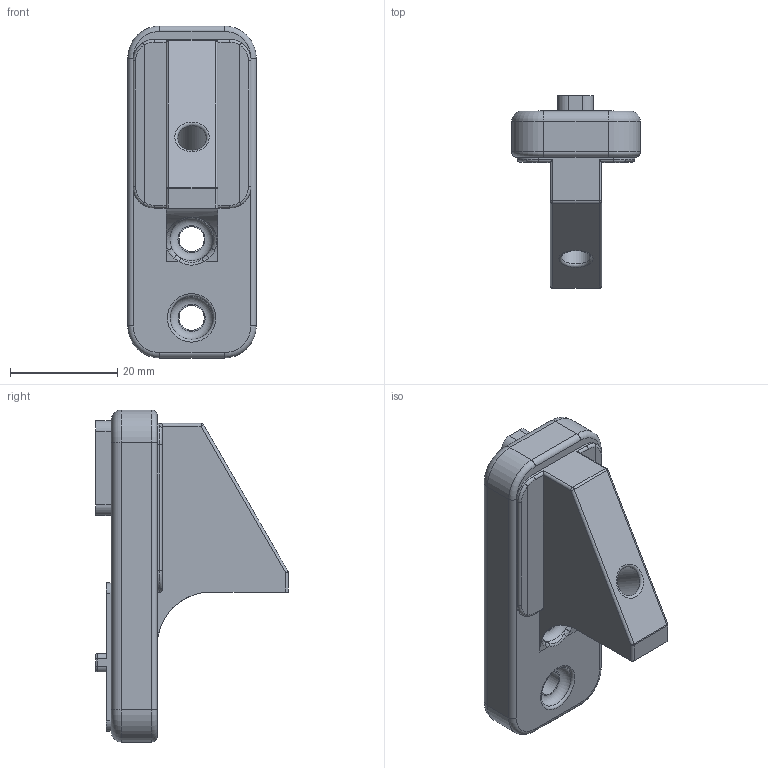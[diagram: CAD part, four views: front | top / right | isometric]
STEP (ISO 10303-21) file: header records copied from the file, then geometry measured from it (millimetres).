
FILE_DESCRIPTION(/* description */ (''),/* implementation_level */ '2;1');
FILE_NAME(/* name */ 'foregrip-adapter-mlok-freeman1337.step',/* time_stamp */ '2021-04-15T20:24:15-07:00',/* author */ (''),/* organization */ (''),/* preprocessor_version */ 'ST-DEVELOPER v18.1',/* originating_system */ 'Autodesk Translation Framework v10.6.0.1341',/* authorisation */ '');
FILE_SCHEMA (('AUTOMOTIVE_DESIGN { 1 0 10303 214 3 1 1 }'));
Length unit declared in the file: millimetre
Products named in the file (1): mlok-adapter
Bounding box: 24 x 35.95 x 62 mm (x, y, z)
Volume: 17848 mm3; surface area: 6291.9 mm2
Topology: 1 solids, 1 shells, 127 faces, 306 edges, 185 vertices
Faces by surface type: cylinder 52, plane 38, torus 22, bspline 11, sphere 4
Full cylindrical faces by diameter (mm): 4.65 x2, 5.41 x1
Entity records: 4258 total; most frequent: CARTESIAN_POINT 1227, DIRECTION 662, ORIENTED_EDGE 612, EDGE_CURVE 306, AXIS2_PLACEMENT_3D 263, VERTEX_POINT 185, LINE 136, VECTOR 136
